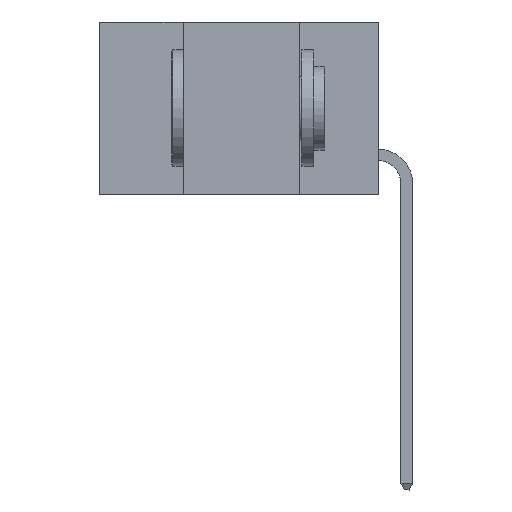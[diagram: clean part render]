
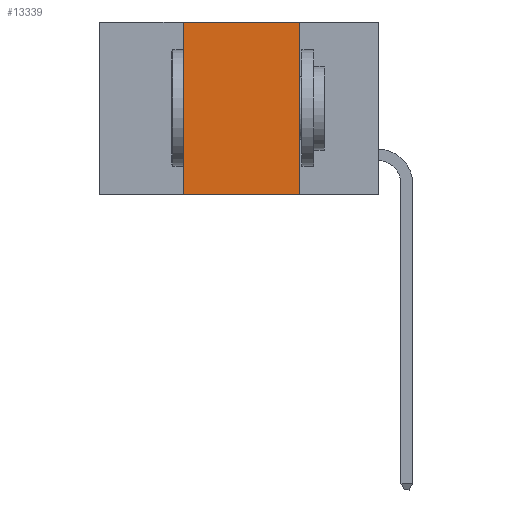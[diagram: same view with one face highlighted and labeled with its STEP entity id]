
A CAD part, left-side view. The second image highlights one B-rep face of the part: STEP entity #13339.
In plain terms, the highlighted planar face has unit normal (-1, 0, 0).
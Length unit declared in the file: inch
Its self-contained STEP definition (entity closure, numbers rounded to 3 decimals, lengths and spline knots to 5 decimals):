
#883 = VERTEX_POINT ( 'NONE', #8708 ) ;
#1046 = LINE ( 'NONE', #5245, #12348 ) ;
#1663 = EDGE_CURVE ( 'NONE', #883, #10999, #10883, .T. ) ;
#1842 = LINE ( 'NONE', #10421, #8023 ) ;
#1895 = EDGE_CURVE ( 'NONE', #2482, #883, #2870, .T. ) ;
#2337 = VERTEX_POINT ( 'NONE', #4925 ) ;
#2454 = CARTESIAN_POINT ( 'NONE',  ( 0., 0.17, -0.37 ) ) ;
#2482 = VERTEX_POINT ( 'NONE', #6193 ) ;
#2870 = LINE ( 'NONE', #3860, #6771 ) ;
#2921 = DIRECTION ( 'NONE',  ( 0., -1., 0. ) ) ;
#3860 = CARTESIAN_POINT ( 'NONE',  ( 0., 0.6, 0. ) ) ;
#4186 = PLANE ( 'NONE',  #9451 ) ;
#4326 = DIRECTION ( 'NONE',  ( 1., 0., 0. ) ) ;
#4370 = DIRECTION ( 'NONE',  ( 0., 0., -1. ) ) ;
#4797 = DIRECTION ( 'NONE',  ( 0., -1., 0. ) ) ;
#4925 = CARTESIAN_POINT ( 'NONE',  ( 0., 0.42, -0.37 ) ) ;
#4950 = ORIENTED_EDGE ( 'NONE', *, *, #10297, .T. ) ;
#5245 = CARTESIAN_POINT ( 'NONE',  ( 0., 0.42, -0.37 ) ) ;
#6193 = CARTESIAN_POINT ( 'NONE',  ( 0., 0.42, 0. ) ) ;
#6771 = VECTOR ( 'NONE', #4797, 39.37008 ) ;
#7335 = ORIENTED_EDGE ( 'NONE', *, *, #10835, .F. ) ;
#8023 = VECTOR ( 'NONE', #2921, 39.37008 ) ;
#8350 = VECTOR ( 'NONE', #4370, 39.37008 ) ;
#8477 = CARTESIAN_POINT ( 'NONE',  ( 0., 0.17, -0.37 ) ) ;
#8528 = ORIENTED_EDGE ( 'NONE', *, *, #1663, .F. ) ;
#8708 = CARTESIAN_POINT ( 'NONE',  ( 0., 0.17, 0. ) ) ;
#9451 = AXIS2_PLACEMENT_3D ( 'NONE', #11842, #4326, #12835 ) ;
#9462 = ORIENTED_EDGE ( 'NONE', *, *, #1895, .F. ) ;
#10297 = EDGE_CURVE ( 'NONE', #2337, #10999, #1842, .T. ) ;
#10421 = CARTESIAN_POINT ( 'NONE',  ( 0., 0.6, -0.37 ) ) ;
#10509 = EDGE_LOOP ( 'NONE', ( #8528, #9462, #7335, #4950 ) ) ;
#10835 = EDGE_CURVE ( 'NONE', #2337, #2482, #1046, .T. ) ;
#10883 = LINE ( 'NONE', #8477, #8350 ) ;
#10999 = VERTEX_POINT ( 'NONE', #2454 ) ;
#11635 = FACE_OUTER_BOUND ( 'NONE', #10509, .T. ) ;
#11842 = CARTESIAN_POINT ( 'NONE',  ( 0., 0.6, 0. ) ) ;
#12348 = VECTOR ( 'NONE', #12890, 39.37008 ) ;
#12835 = DIRECTION ( 'NONE',  ( 0., 0., -1. ) ) ;
#12890 = DIRECTION ( 'NONE',  ( 0., 0., 1. ) ) ;
#13339 = ADVANCED_FACE ( 'NONE', ( #11635 ), #4186, .F. ) ;
